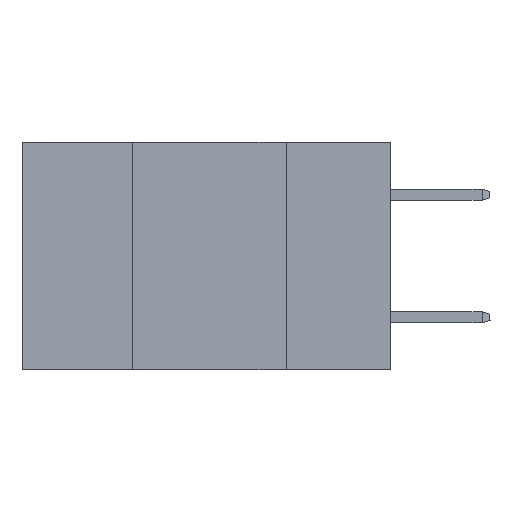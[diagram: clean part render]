
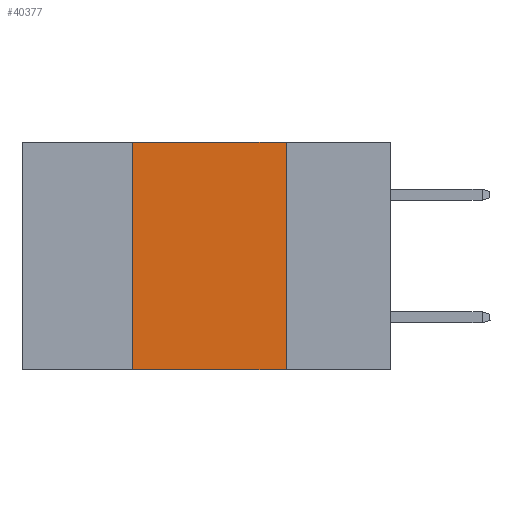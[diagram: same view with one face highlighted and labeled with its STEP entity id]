
A CAD part, left-side view. The second image highlights one B-rep face of the part: STEP entity #40377.
In plain terms, the highlighted planar face has unit normal (-1, 0, 0).
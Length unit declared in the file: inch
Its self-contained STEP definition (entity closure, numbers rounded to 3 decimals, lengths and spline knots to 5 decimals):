
#460 = CARTESIAN_POINT ( 'NONE',  ( 0., 0.6, 0. ) ) ;
#676 = VECTOR ( 'NONE', #22899, 39.37008 ) ;
#988 = EDGE_CURVE ( 'NONE', #4765, #13994, #29175, .T. ) ;
#3235 = PLANE ( 'NONE',  #30877 ) ;
#4765 = VERTEX_POINT ( 'NONE', #21487 ) ;
#6020 = ORIENTED_EDGE ( 'NONE', *, *, #37566, .F. ) ;
#6173 = FACE_OUTER_BOUND ( 'NONE', #16369, .T. ) ;
#6479 = ORIENTED_EDGE ( 'NONE', *, *, #24858, .F. ) ;
#8656 = VECTOR ( 'NONE', #26225, 39.37008 ) ;
#11574 = ORIENTED_EDGE ( 'NONE', *, *, #17711, .T. ) ;
#12665 = CARTESIAN_POINT ( 'NONE',  ( 0., 0.6, 0. ) ) ;
#13271 = DIRECTION ( 'NONE',  ( 1., 0., 0. ) ) ;
#13443 = LINE ( 'NONE', #22898, #8656 ) ;
#13994 = VERTEX_POINT ( 'NONE', #31246 ) ;
#14694 = CARTESIAN_POINT ( 'NONE',  ( 0., 0.17, -0.37 ) ) ;
#15456 = LINE ( 'NONE', #28245, #36448 ) ;
#16130 = CARTESIAN_POINT ( 'NONE',  ( 0., 0.42, -0.37 ) ) ;
#16369 = EDGE_LOOP ( 'NONE', ( #6479, #37704, #6020, #11574 ) ) ;
#17203 = VERTEX_POINT ( 'NONE', #16130 ) ;
#17711 = EDGE_CURVE ( 'NONE', #17203, #37375, #15456, .T. ) ;
#21487 = CARTESIAN_POINT ( 'NONE',  ( 0., 0.42, 0. ) ) ;
#22898 = CARTESIAN_POINT ( 'NONE',  ( 0., 0.17, 0. ) ) ;
#22899 = DIRECTION ( 'NONE',  ( 0., -1., 0. ) ) ;
#24858 = EDGE_CURVE ( 'NONE', #13994, #37375, #13443, .T. ) ;
#26225 = DIRECTION ( 'NONE',  ( 0., 0., -1. ) ) ;
#28245 = CARTESIAN_POINT ( 'NONE',  ( 0., 0.6, -0.37 ) ) ;
#28789 = DIRECTION ( 'NONE',  ( 0., 0., -1. ) ) ;
#29175 = LINE ( 'NONE', #460, #676 ) ;
#30877 = AXIS2_PLACEMENT_3D ( 'NONE', #12665, #13271, #28789 ) ;
#31246 = CARTESIAN_POINT ( 'NONE',  ( 0., 0.17, 0. ) ) ;
#32143 = VECTOR ( 'NONE', #34394, 39.37008 ) ;
#34180 = LINE ( 'NONE', #37948, #32143 ) ;
#34394 = DIRECTION ( 'NONE',  ( 0., 0., 1. ) ) ;
#36448 = VECTOR ( 'NONE', #38073, 39.37008 ) ;
#37375 = VERTEX_POINT ( 'NONE', #14694 ) ;
#37566 = EDGE_CURVE ( 'NONE', #17203, #4765, #34180, .T. ) ;
#37704 = ORIENTED_EDGE ( 'NONE', *, *, #988, .F. ) ;
#37948 = CARTESIAN_POINT ( 'NONE',  ( 0., 0.42, 0. ) ) ;
#38073 = DIRECTION ( 'NONE',  ( 0., -1., 0. ) ) ;
#40377 = ADVANCED_FACE ( 'NONE', ( #6173 ), #3235, .F. ) ;
